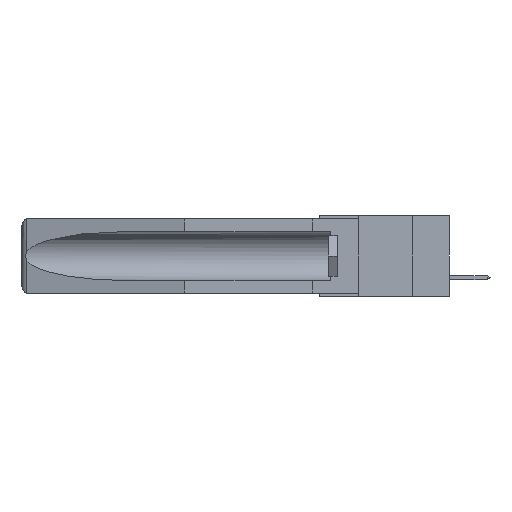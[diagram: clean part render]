
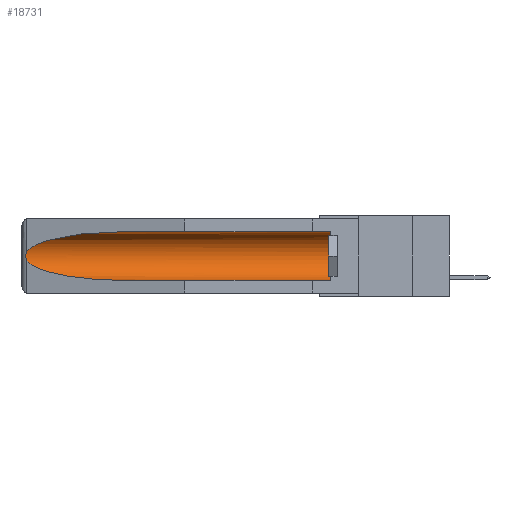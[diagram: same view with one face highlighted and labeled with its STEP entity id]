
A CAD part, left-side view. The second image highlights one B-rep face of the part: STEP entity #18731.
In plain terms, the highlighted cylindrical face has radius 2.857 mm (diameter 5.715 mm), a partial arc.
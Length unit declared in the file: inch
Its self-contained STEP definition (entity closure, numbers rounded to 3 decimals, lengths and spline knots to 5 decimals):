
#394 = EDGE_CURVE ( 'NONE', #1928, #408, #11795, .T. ) ;
#408 = VERTEX_POINT ( 'NONE', #15322 ) ;
#566 = CARTESIAN_POINT ( 'NONE',  ( 0.26537, 1.52718, -0.19328 ) ) ;
#1145 = DIRECTION ( 'NONE',  ( 0., 1., 0. ) ) ;
#1541 = VERTEX_POINT ( 'NONE', #5670 ) ;
#1634 = EDGE_CURVE ( 'NONE', #1541, #26516, #11721, .T. ) ;
#1788 = AXIS2_PLACEMENT_3D ( 'NONE', #8389, #16624, #14567 ) ;
#1928 = VERTEX_POINT ( 'NONE', #10722 ) ;
#2067 = VERTEX_POINT ( 'NONE', #3624 ) ;
#2364 = ORIENTED_EDGE ( 'NONE', *, *, #25893, .T. ) ;
#2566 = EDGE_LOOP ( 'NONE', ( #13509, #11054, #5927, #6102, #2364, #19809 ) ) ;
#2707 = CARTESIAN_POINT ( 'NONE',  ( 0.26537, 1.52718, -0.19328 ) ) ;
#3198 = AXIS2_PLACEMENT_3D ( 'NONE', #17904, #1145, #7436 ) ;
#3598 =( BOUNDED_CURVE ( )  B_SPLINE_CURVE ( 3, ( #23357, #14988, #5005, #17200 ),
 .UNSPECIFIED., .F., .F. ) 
 B_SPLINE_CURVE_WITH_KNOTS ( ( 4, 4 ),
 ( 4.71239, 6.08839 ),
 .UNSPECIFIED. ) 
 CURVE ( )  GEOMETRIC_REPRESENTATION_ITEM ( )  RATIONAL_B_SPLINE_CURVE ( ( 1., 0.848, 0.848, 1. ) ) 
 REPRESENTATION_ITEM ( '' )  );
#3613 = EDGE_CURVE ( 'NONE', #26516, #2067, #3598, .T. ) ;
#3624 = CARTESIAN_POINT ( 'NONE',  ( 0.26537, 1.52718, -0.14972 ) ) ;
#4917 = VERTEX_POINT ( 'NONE', #566 ) ;
#5005 = CARTESIAN_POINT ( 'NONE',  ( 0.25451, 1.48313, -0.09465 ) ) ;
#5058 = CARTESIAN_POINT ( 'NONE',  ( 0.25451, 1.48313, -0.24835 ) ) ;
#5486 = CARTESIAN_POINT ( 'NONE',  ( 0.26537, 1.52718, -0.19328 ) ) ;
#5661 = CARTESIAN_POINT ( 'NONE',  ( 0.26654, 1.53092, -0.15636 ) ) ;
#5670 = CARTESIAN_POINT ( 'NONE',  ( 0.155, 0.126, -0.059 ) ) ;
#5743 = CARTESIAN_POINT ( 'NONE',  ( 0.2675, 1.53308, -0.17534 ) ) ;
#5927 = ORIENTED_EDGE ( 'NONE', *, *, #9765, .T. ) ;
#6102 = ORIENTED_EDGE ( 'NONE', *, *, #394, .F. ) ;
#7436 = DIRECTION ( 'NONE',  ( 0., 0., 1. ) ) ;
#7657 = EDGE_CURVE ( 'NONE', #2067, #4917, #9210, .T. ) ;
#7807 = CARTESIAN_POINT ( 'NONE',  ( 0.26597, 1.5296, -0.19026 ) ) ;
#8389 = CARTESIAN_POINT ( 'NONE',  ( 0.155, 0.126, -0.1715 ) ) ;
#9106 = CIRCLE ( 'NONE', #1788, 0.1125 ) ;
#9210 = B_SPLINE_CURVE_WITH_KNOTS ( 'NONE', 3,
 ( #19721, #13812, #5661, #15982, #19981, #5743, #26068, #22036, #7807, #5486 ),
 .UNSPECIFIED., .F., .F.,
 ( 4, 2, 2, 2, 4 ),
 ( 0., 0.00029, 0.00058, 0.00087, 0.00117 ),
 .UNSPECIFIED. ) ;
#9765 = EDGE_CURVE ( 'NONE', #4917, #408, #24271, .T. ) ;
#10126 = CYLINDRICAL_SURFACE ( 'NONE', #3198, 0.1125 ) ;
#10131 = DIRECTION ( 'NONE',  ( 0., 1., 0. ) ) ;
#10722 = CARTESIAN_POINT ( 'NONE',  ( 0.155, 0.126, -0.284 ) ) ;
#11054 = ORIENTED_EDGE ( 'NONE', *, *, #7657, .T. ) ;
#11241 = CARTESIAN_POINT ( 'NONE',  ( 0.155, -0.30754, -0.284 ) ) ;
#11243 = CARTESIAN_POINT ( 'NONE',  ( 0.21114, 1.30732, -0.284 ) ) ;
#11721 = LINE ( 'NONE', #22394, #25475 ) ;
#11795 = LINE ( 'NONE', #11241, #24259 ) ;
#13039 = CARTESIAN_POINT ( 'NONE',  ( 0.155, 1.07973, -0.284 ) ) ;
#13509 = ORIENTED_EDGE ( 'NONE', *, *, #3613, .T. ) ;
#13812 = CARTESIAN_POINT ( 'NONE',  ( 0.26597, 1.52961, -0.15275 ) ) ;
#14567 = DIRECTION ( 'NONE',  ( 0., 0., 1. ) ) ;
#14988 = CARTESIAN_POINT ( 'NONE',  ( 0.21114, 1.30732, -0.059 ) ) ;
#15322 = CARTESIAN_POINT ( 'NONE',  ( 0.155, 1.07973, -0.284 ) ) ;
#15982 = CARTESIAN_POINT ( 'NONE',  ( 0.2673, 1.5327, -0.16383 ) ) ;
#16529 = FACE_OUTER_BOUND ( 'NONE', #2566, .T. ) ;
#16624 = DIRECTION ( 'NONE',  ( 0., -1., 0. ) ) ;
#17200 = CARTESIAN_POINT ( 'NONE',  ( 0.26537, 1.52718, -0.14972 ) ) ;
#17904 = CARTESIAN_POINT ( 'NONE',  ( 0.155, -0.30754, -0.1715 ) ) ;
#18731 = ADVANCED_FACE ( 'NONE', ( #16529 ), #10126, .F. ) ;
#19721 = CARTESIAN_POINT ( 'NONE',  ( 0.26537, 1.52718, -0.14972 ) ) ;
#19809 = ORIENTED_EDGE ( 'NONE', *, *, #1634, .T. ) ;
#19981 = CARTESIAN_POINT ( 'NONE',  ( 0.2675, 1.53308, -0.16763 ) ) ;
#21267 = DIRECTION ( 'NONE',  ( 0., 1., 0. ) ) ;
#21326 = CARTESIAN_POINT ( 'NONE',  ( 0.155, 1.07973, -0.059 ) ) ;
#22036 = CARTESIAN_POINT ( 'NONE',  ( 0.26655, 1.53094, -0.18657 ) ) ;
#22394 = CARTESIAN_POINT ( 'NONE',  ( 0.155, -0.30754, -0.059 ) ) ;
#23357 = CARTESIAN_POINT ( 'NONE',  ( 0.155, 1.07973, -0.059 ) ) ;
#24259 = VECTOR ( 'NONE', #21267, 39.37008 ) ;
#24271 =( BOUNDED_CURVE ( )  B_SPLINE_CURVE ( 3, ( #2707, #5058, #11243, #13039 ),
 .UNSPECIFIED., .F., .F. ) 
 B_SPLINE_CURVE_WITH_KNOTS ( ( 4, 4 ),
 ( 0.1948, 1.5708 ),
 .UNSPECIFIED. ) 
 CURVE ( )  GEOMETRIC_REPRESENTATION_ITEM ( )  RATIONAL_B_SPLINE_CURVE ( ( 1., 0.848, 0.848, 1. ) ) 
 REPRESENTATION_ITEM ( '' )  );
#25475 = VECTOR ( 'NONE', #10131, 39.37008 ) ;
#25893 = EDGE_CURVE ( 'NONE', #1928, #1541, #9106, .T. ) ;
#26068 = CARTESIAN_POINT ( 'NONE',  ( 0.2673, 1.53269, -0.17917 ) ) ;
#26516 = VERTEX_POINT ( 'NONE', #21326 ) ;
